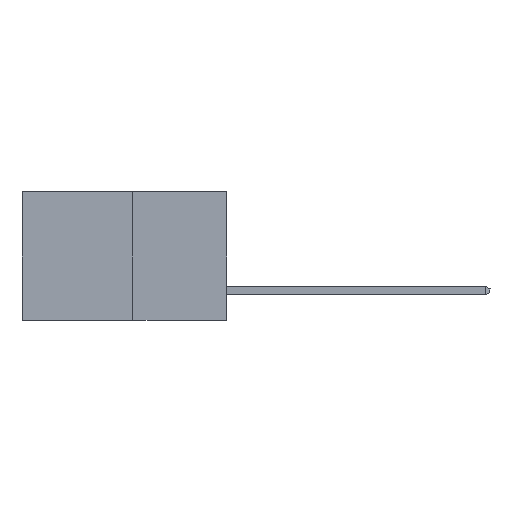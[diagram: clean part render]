
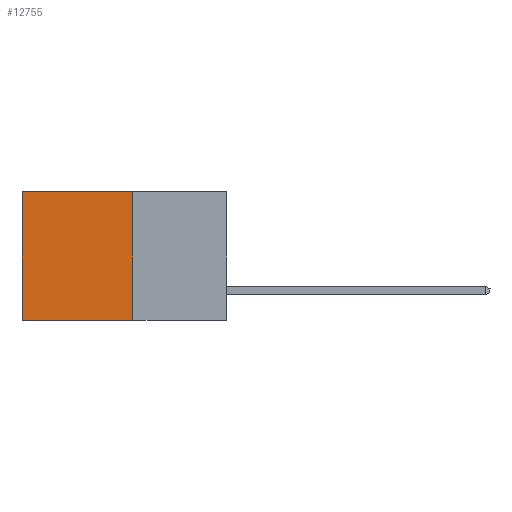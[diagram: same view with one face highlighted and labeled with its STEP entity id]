
A CAD part, left-side view. The second image highlights one B-rep face of the part: STEP entity #12755.
In plain terms, the highlighted planar face has unit normal (-1, 0, 0).
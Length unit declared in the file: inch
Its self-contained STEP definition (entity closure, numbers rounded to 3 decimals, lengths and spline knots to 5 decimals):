
#2010 = VERTEX_POINT ( 'NONE', #13250 ) ;
#2689 = VECTOR ( 'NONE', #12162, 39.37008 ) ;
#3056 = EDGE_CURVE ( 'NONE', #4655, #2010, #6198, .T. ) ;
#3348 = AXIS2_PLACEMENT_3D ( 'NONE', #11656, #4612, #12797 ) ;
#3418 = CARTESIAN_POINT ( 'NONE',  ( 0.277, 0.27, 0. ) ) ;
#4123 = EDGE_LOOP ( 'NONE', ( #7625, #11291, #12186, #6701 ) ) ;
#4612 = DIRECTION ( 'NONE',  ( 1., 0., 0. ) ) ;
#4655 = VERTEX_POINT ( 'NONE', #15669 ) ;
#5134 = EDGE_CURVE ( 'NONE', #13819, #7745, #9674, .T. ) ;
#5141 = VECTOR ( 'NONE', #9934, 39.37008 ) ;
#5155 = CARTESIAN_POINT ( 'NONE',  ( 0.277, 0.27, -0.37 ) ) ;
#5480 = VECTOR ( 'NONE', #7261, 39.37008 ) ;
#6198 = LINE ( 'NONE', #12975, #2689 ) ;
#6701 = ORIENTED_EDGE ( 'NONE', *, *, #15398, .T. ) ;
#7261 = DIRECTION ( 'NONE',  ( 0., 1., 0. ) ) ;
#7625 = ORIENTED_EDGE ( 'NONE', *, *, #5134, .T. ) ;
#7745 = VERTEX_POINT ( 'NONE', #9861 ) ;
#8598 = LINE ( 'NONE', #3418, #5480 ) ;
#9000 = EDGE_CURVE ( 'NONE', #2010, #7745, #11351, .T. ) ;
#9215 = VECTOR ( 'NONE', #15655, 39.37008 ) ;
#9674 = LINE ( 'NONE', #15640, #9215 ) ;
#9861 = CARTESIAN_POINT ( 'NONE',  ( 0.277, 0.59, -0.37 ) ) ;
#9934 = DIRECTION ( 'NONE',  ( 0., 1., 0. ) ) ;
#11259 = CARTESIAN_POINT ( 'NONE',  ( 0.277, 0.59, 0. ) ) ;
#11291 = ORIENTED_EDGE ( 'NONE', *, *, #9000, .F. ) ;
#11351 = LINE ( 'NONE', #5155, #5141 ) ;
#11656 = CARTESIAN_POINT ( 'NONE',  ( 0.277, 0.27, -0.37 ) ) ;
#11903 = FACE_OUTER_BOUND ( 'NONE', #4123, .T. ) ;
#12162 = DIRECTION ( 'NONE',  ( 0., 0., -1. ) ) ;
#12186 = ORIENTED_EDGE ( 'NONE', *, *, #3056, .F. ) ;
#12750 = PLANE ( 'NONE',  #3348 ) ;
#12755 = ADVANCED_FACE ( 'NONE', ( #11903 ), #12750, .F. ) ;
#12797 = DIRECTION ( 'NONE',  ( 0., 0., -1. ) ) ;
#12975 = CARTESIAN_POINT ( 'NONE',  ( 0.277, 0.27, -0.37 ) ) ;
#13250 = CARTESIAN_POINT ( 'NONE',  ( 0.277, 0.27, -0.37 ) ) ;
#13819 = VERTEX_POINT ( 'NONE', #11259 ) ;
#15398 = EDGE_CURVE ( 'NONE', #4655, #13819, #8598, .T. ) ;
#15640 = CARTESIAN_POINT ( 'NONE',  ( 0.277, 0.59, -0.37 ) ) ;
#15655 = DIRECTION ( 'NONE',  ( 0., 0., -1. ) ) ;
#15669 = CARTESIAN_POINT ( 'NONE',  ( 0.277, 0.27, 0. ) ) ;
